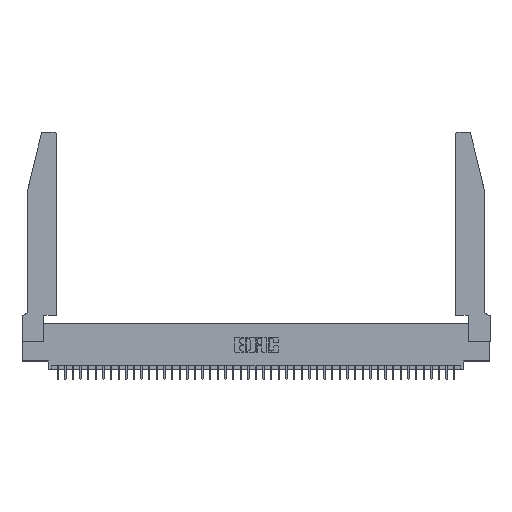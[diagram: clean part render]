
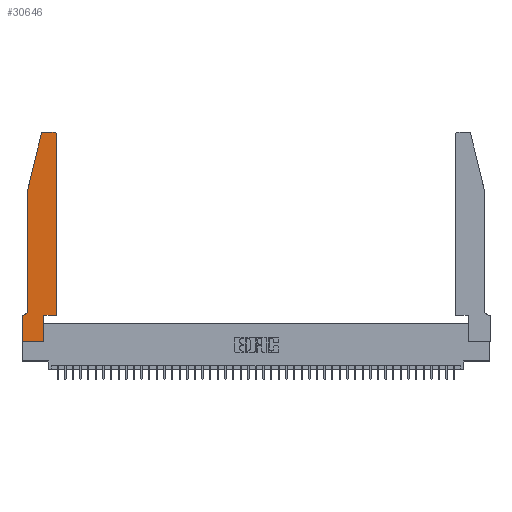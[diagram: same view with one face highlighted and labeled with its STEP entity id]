
A CAD part, top view. The second image highlights one B-rep face of the part: STEP entity #30646.
In plain terms, the highlighted planar face has unit normal (0, 0, 1).
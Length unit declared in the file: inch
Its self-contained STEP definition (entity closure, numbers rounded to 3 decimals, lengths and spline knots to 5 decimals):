
#960 = DIRECTION ( 'NONE',  ( 1., 0., 0. ) ) ;
#1268 = CARTESIAN_POINT ( 'NONE',  ( 0.0755, 2., 0.37 ) ) ;
#1741 = ORIENTED_EDGE ( 'NONE', *, *, #15799, .T. ) ;
#2004 = CARTESIAN_POINT ( 'NONE',  ( 0.4505, 0.35, 0.37 ) ) ;
#2268 = DIRECTION ( 'NONE',  ( 0., -1., 0. ) ) ;
#3362 = CARTESIAN_POINT ( 'NONE',  ( 0., 0.35, 0.37 ) ) ;
#3802 = LINE ( 'NONE', #25012, #5753 ) ;
#4146 = LINE ( 'NONE', #16153, #38191 ) ;
#5018 = LINE ( 'NONE', #8218, #31543 ) ;
#5753 = VECTOR ( 'NONE', #28448, 39.37008 ) ;
#6265 = CARTESIAN_POINT ( 'NONE',  ( 0.4505, 0.35, 0.37 ) ) ;
#6317 = CARTESIAN_POINT ( 'NONE',  ( 0.0755, 0.42, 0.37 ) ) ;
#6428 = VERTEX_POINT ( 'NONE', #39742 ) ;
#6543 = CARTESIAN_POINT ( 'NONE',  ( 0.25487, 2.72718, 0.37 ) ) ;
#6710 = CARTESIAN_POINT ( 'NONE',  ( 0.0755, 2., 0.37 ) ) ;
#7126 = VERTEX_POINT ( 'NONE', #6543 ) ;
#7233 = ORIENTED_EDGE ( 'NONE', *, *, #16706, .T. ) ;
#7633 = VECTOR ( 'NONE', #18416, 39.37008 ) ;
#8082 = DIRECTION ( 'NONE',  ( 0., 0., -1. ) ) ;
#8218 = CARTESIAN_POINT ( 'NONE',  ( 0.4505, 0.35, 0.37 ) ) ;
#8784 = DIRECTION ( 'NONE',  ( 0., -1., 0. ) ) ;
#9042 = VECTOR ( 'NONE', #8784, 39.37008 ) ;
#9141 = VERTEX_POINT ( 'NONE', #6265 ) ;
#10677 = ORIENTED_EDGE ( 'NONE', *, *, #12710, .T. ) ;
#11895 = CARTESIAN_POINT ( 'NONE',  ( 0.284, 2.72, 0.37 ) ) ;
#12095 = DIRECTION ( 'NONE',  ( -0.239, -0.971, 0. ) ) ;
#12333 = VERTEX_POINT ( 'NONE', #15723 ) ;
#12710 = EDGE_CURVE ( 'NONE', #6428, #9141, #5018, .T. ) ;
#12835 = VERTEX_POINT ( 'NONE', #40714 ) ;
#13100 = AXIS2_PLACEMENT_3D ( 'NONE', #11895, #14893, #960 ) ;
#13528 = CARTESIAN_POINT ( 'NONE',  ( 0.2605, 2.75, 0.37 ) ) ;
#14280 = ORIENTED_EDGE ( 'NONE', *, *, #24770, .T. ) ;
#14893 = DIRECTION ( 'NONE',  ( 0., 0., 1. ) ) ;
#15309 = CIRCLE ( 'NONE', #28459, 0.03 ) ;
#15723 = CARTESIAN_POINT ( 'NONE',  ( 0.2865, 0., 0.37 ) ) ;
#15799 = EDGE_CURVE ( 'NONE', #41744, #12333, #3802, .T. ) ;
#15802 = DIRECTION ( 'NONE',  ( -1., 0., 0. ) ) ;
#16065 = VERTEX_POINT ( 'NONE', #6317 ) ;
#16153 = CARTESIAN_POINT ( 'NONE',  ( 0.2865, 0.35, 0.37 ) ) ;
#16358 = EDGE_CURVE ( 'NONE', #12333, #6428, #4146, .T. ) ;
#16706 = EDGE_CURVE ( 'NONE', #17161, #16065, #25648, .T. ) ;
#16784 = VERTEX_POINT ( 'NONE', #3362 ) ;
#17161 = VERTEX_POINT ( 'NONE', #6710 ) ;
#18416 = DIRECTION ( 'NONE',  ( 0., 1., 0. ) ) ;
#18482 = ORIENTED_EDGE ( 'NONE', *, *, #19713, .T. ) ;
#18649 = VECTOR ( 'NONE', #2268, 39.37008 ) ;
#18989 = CARTESIAN_POINT ( 'NONE',  ( 0.0055, 0.42, 0.37 ) ) ;
#19097 = CARTESIAN_POINT ( 'NONE',  ( 0.0055, 0.35, 0.37 ) ) ;
#19101 = CARTESIAN_POINT ( 'NONE',  ( 0.4505, 2.72, 0.37 ) ) ;
#19120 = DIRECTION ( 'NONE',  ( 1., 0., 0. ) ) ;
#19306 = LINE ( 'NONE', #2004, #7633 ) ;
#19357 = LINE ( 'NONE', #30318, #28879 ) ;
#19713 = EDGE_CURVE ( 'NONE', #16065, #40371, #25805, .T. ) ;
#19796 = LINE ( 'NONE', #33751, #18649 ) ;
#19865 = LINE ( 'NONE', #29493, #42982 ) ;
#19912 = ORIENTED_EDGE ( 'NONE', *, *, #20005, .T. ) ;
#20005 = EDGE_CURVE ( 'NONE', #9141, #43246, #19306, .T. ) ;
#22345 = EDGE_CURVE ( 'NONE', #7126, #17161, #19357, .T. ) ;
#22829 = CARTESIAN_POINT ( 'NONE',  ( 0.4205, 2.72, 0.37 ) ) ;
#23321 = PLANE ( 'NONE',  #35225 ) ;
#24020 = CIRCLE ( 'NONE', #13100, 0.03 ) ;
#24770 = EDGE_CURVE ( 'NONE', #44460, #12835, #44762, .T. ) ;
#24946 = EDGE_LOOP ( 'NONE', ( #14280, #42670, #42442, #7233, #18482, #40731, #28546, #1741, #30065, #10677, #19912, #35504 ) ) ;
#25012 = CARTESIAN_POINT ( 'NONE',  ( 0., 0., 0.37 ) ) ;
#25648 = LINE ( 'NONE', #1268, #9042 ) ;
#25805 = CIRCLE ( 'NONE', #36770, 0.07 ) ;
#25853 = DIRECTION ( 'NONE',  ( -1., 0., 0. ) ) ;
#27428 = CARTESIAN_POINT ( 'NONE',  ( 0.4205, 2.75, 0.37 ) ) ;
#28448 = DIRECTION ( 'NONE',  ( 1., 0., 0. ) ) ;
#28459 = AXIS2_PLACEMENT_3D ( 'NONE', #22829, #39987, #39763 ) ;
#28481 = EDGE_CURVE ( 'NONE', #40371, #16784, #19865, .T. ) ;
#28546 = ORIENTED_EDGE ( 'NONE', *, *, #41039, .T. ) ;
#28879 = VECTOR ( 'NONE', #12095, 39.37008 ) ;
#28948 = EDGE_CURVE ( 'NONE', #12835, #7126, #24020, .T. ) ;
#29493 = CARTESIAN_POINT ( 'NONE',  ( 0.0755, 0.35, 0.37 ) ) ;
#30065 = ORIENTED_EDGE ( 'NONE', *, *, #16358, .T. ) ;
#30318 = CARTESIAN_POINT ( 'NONE',  ( 0.0755, 2., 0.37 ) ) ;
#30412 = FACE_OUTER_BOUND ( 'NONE', #24946, .T. ) ;
#30646 = ADVANCED_FACE ( 'NONE', ( #30412 ), #23321, .T. ) ;
#31543 = VECTOR ( 'NONE', #19120, 39.37008 ) ;
#32178 = EDGE_CURVE ( 'NONE', #43246, #44460, #15309, .T. ) ;
#33743 = DIRECTION ( 'NONE',  ( 0., 1., 0. ) ) ;
#33751 = CARTESIAN_POINT ( 'NONE',  ( 0., 0., 0.37 ) ) ;
#33853 = CARTESIAN_POINT ( 'NONE',  ( 0., 0.35, 0.37 ) ) ;
#35158 = DIRECTION ( 'NONE',  ( 0., 0., 1. ) ) ;
#35225 = AXIS2_PLACEMENT_3D ( 'NONE', #33853, #35158, #44332 ) ;
#35504 = ORIENTED_EDGE ( 'NONE', *, *, #32178, .T. ) ;
#36770 = AXIS2_PLACEMENT_3D ( 'NONE', #18989, #8082, #25853 ) ;
#37680 = VECTOR ( 'NONE', #41575, 39.37008 ) ;
#38191 = VECTOR ( 'NONE', #33743, 39.37008 ) ;
#38783 = CARTESIAN_POINT ( 'NONE',  ( 0., 0., 0.37 ) ) ;
#39742 = CARTESIAN_POINT ( 'NONE',  ( 0.2865, 0.35, 0.37 ) ) ;
#39763 = DIRECTION ( 'NONE',  ( 1., 0., 0. ) ) ;
#39987 = DIRECTION ( 'NONE',  ( 0., 0., 1. ) ) ;
#40371 = VERTEX_POINT ( 'NONE', #19097 ) ;
#40714 = CARTESIAN_POINT ( 'NONE',  ( 0.284, 2.75, 0.37 ) ) ;
#40731 = ORIENTED_EDGE ( 'NONE', *, *, #28481, .T. ) ;
#41039 = EDGE_CURVE ( 'NONE', #16784, #41744, #19796, .T. ) ;
#41575 = DIRECTION ( 'NONE',  ( -1., 0., 0. ) ) ;
#41744 = VERTEX_POINT ( 'NONE', #38783 ) ;
#42442 = ORIENTED_EDGE ( 'NONE', *, *, #22345, .T. ) ;
#42670 = ORIENTED_EDGE ( 'NONE', *, *, #28948, .T. ) ;
#42982 = VECTOR ( 'NONE', #15802, 39.37008 ) ;
#43246 = VERTEX_POINT ( 'NONE', #19101 ) ;
#44332 = DIRECTION ( 'NONE',  ( 1., 0., 0. ) ) ;
#44460 = VERTEX_POINT ( 'NONE', #27428 ) ;
#44762 = LINE ( 'NONE', #13528, #37680 ) ;
